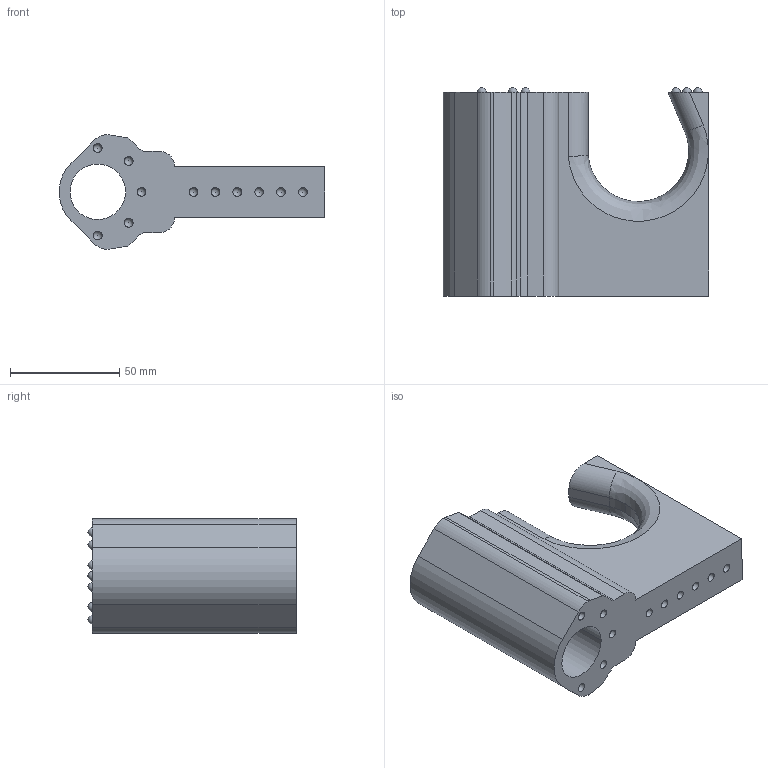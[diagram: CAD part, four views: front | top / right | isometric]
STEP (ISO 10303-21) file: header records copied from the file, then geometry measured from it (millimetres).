
FILE_DESCRIPTION (( 'STEP AP214' ), '1' );
FILE_NAME ('Stock Front.STEP', '2013-06-24T22:50:04', ( 'Asher' ), ( '' ), 'SwSTEP 2.0', 'SolidWorks 2013', '' );
FILE_SCHEMA (( 'AUTOMOTIVE_DESIGN' ));
Length unit declared in the file: millimetre
Products named in the file (1): Stock Front
Bounding box: 121.38 x 95.25 x 52.5 mm (x, y, z)
Volume: 244592.1 mm3; surface area: 39893.2 mm2
Topology: 1 solids, 1 shells, 65 faces, 214 edges, 144 vertices
Faces by surface type: sphere 27, cylinder 21, plane 14, bspline 3
Entity records: 2384 total; most frequent: CARTESIAN_POINT 692, DIRECTION 367, ORIENTED_EDGE 320, EDGE_CURVE 160, AXIS2_PLACEMENT_3D 155, VERTEX_POINT 124, EDGE_LOOP 94, CIRCLE 92
